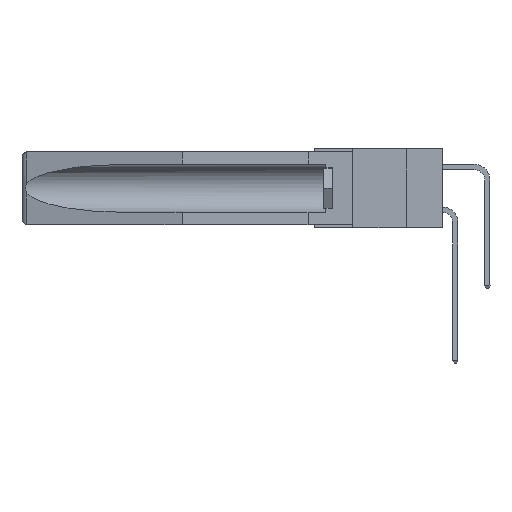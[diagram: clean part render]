
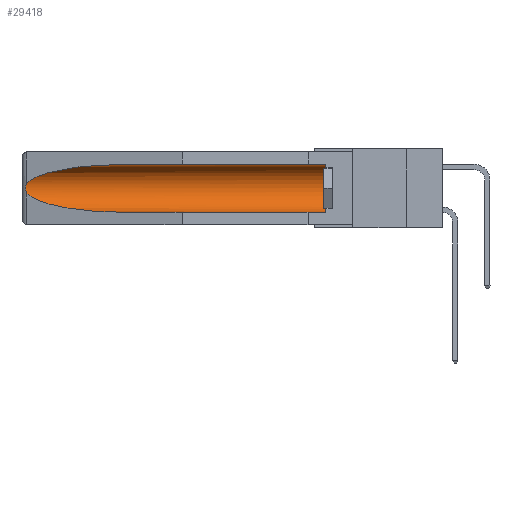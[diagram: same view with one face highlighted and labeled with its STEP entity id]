
A CAD part, left-side view. The second image highlights one B-rep face of the part: STEP entity #29418.
In plain terms, the highlighted cylindrical face has radius 2.857 mm (diameter 5.715 mm), a partial arc.
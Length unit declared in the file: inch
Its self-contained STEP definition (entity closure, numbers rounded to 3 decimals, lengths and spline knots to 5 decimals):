
#142 = EDGE_CURVE ( 'NONE', #16310, #8320, #24778, .T. ) ;
#195 = CARTESIAN_POINT ( 'NONE',  ( 0.21114, 1.30732, -0.059 ) ) ;
#409 = DIRECTION ( 'NONE',  ( 0., 0., 1. ) ) ;
#1260 = ORIENTED_EDGE ( 'NONE', *, *, #14060, .T. ) ;
#1483 = VERTEX_POINT ( 'NONE', #27589 ) ;
#1517 = CARTESIAN_POINT ( 'NONE',  ( 0.26537, 1.52718, -0.14972 ) ) ;
#1583 = DIRECTION ( 'NONE',  ( 0., 0., 1. ) ) ;
#1936 = CARTESIAN_POINT ( 'NONE',  ( 0.155, -0.30754, -0.284 ) ) ;
#1953 = CARTESIAN_POINT ( 'NONE',  ( 0.26537, 1.52718, -0.19328 ) ) ;
#2326 = VERTEX_POINT ( 'NONE', #5657 ) ;
#2421 = CARTESIAN_POINT ( 'NONE',  ( 0.155, -0.30754, -0.1715 ) ) ;
#5568 = CYLINDRICAL_SURFACE ( 'NONE', #19323, 0.1125 ) ;
#5657 = CARTESIAN_POINT ( 'NONE',  ( 0.155, 1.07973, -0.059 ) ) ;
#6466 = CARTESIAN_POINT ( 'NONE',  ( 0.25451, 1.48313, -0.09465 ) ) ;
#7957 = EDGE_CURVE ( 'NONE', #2326, #8256, #28995, .T. ) ;
#8209 = DIRECTION ( 'NONE',  ( 0., 1., 0. ) ) ;
#8256 = VERTEX_POINT ( 'NONE', #28920 ) ;
#8320 = VERTEX_POINT ( 'NONE', #12853 ) ;
#8803 = CARTESIAN_POINT ( 'NONE',  ( 0.2675, 1.53308, -0.17534 ) ) ;
#8817 = EDGE_CURVE ( 'NONE', #27200, #2326, #30827, .T. ) ;
#8905 = DIRECTION ( 'NONE',  ( 0., 1., 0. ) ) ;
#9609 = LINE ( 'NONE', #1936, #17907 ) ;
#9870 = DIRECTION ( 'NONE',  ( 0., 1., 0. ) ) ;
#10989 = EDGE_CURVE ( 'NONE', #1483, #27200, #17435, .T. ) ;
#10995 = CARTESIAN_POINT ( 'NONE',  ( 0.26655, 1.53094, -0.18657 ) ) ;
#11967 = FACE_OUTER_BOUND ( 'NONE', #29376, .T. ) ;
#12731 = CARTESIAN_POINT ( 'NONE',  ( 0.155, -0.30754, -0.059 ) ) ;
#12853 = CARTESIAN_POINT ( 'NONE',  ( 0.155, 1.07973, -0.284 ) ) ;
#14060 = EDGE_CURVE ( 'NONE', #8256, #16310, #20357, .T. ) ;
#15613 = CARTESIAN_POINT ( 'NONE',  ( 0.2673, 1.53269, -0.17917 ) ) ;
#15722 = CARTESIAN_POINT ( 'NONE',  ( 0.26597, 1.52961, -0.15275 ) ) ;
#16310 = VERTEX_POINT ( 'NONE', #1953 ) ;
#16503 = ORIENTED_EDGE ( 'NONE', *, *, #7957, .T. ) ;
#17119 = CARTESIAN_POINT ( 'NONE',  ( 0.155, 1.07973, -0.284 ) ) ;
#17360 = AXIS2_PLACEMENT_3D ( 'NONE', #20647, #27847, #1583 ) ;
#17435 = CIRCLE ( 'NONE', #17360, 0.1125 ) ;
#17907 = VECTOR ( 'NONE', #8905, 39.37008 ) ;
#18257 = CARTESIAN_POINT ( 'NONE',  ( 0.26537, 1.52718, -0.19328 ) ) ;
#18351 = ORIENTED_EDGE ( 'NONE', *, *, #10989, .T. ) ;
#18420 = VECTOR ( 'NONE', #8209, 39.37008 ) ;
#19200 = CARTESIAN_POINT ( 'NONE',  ( 0.155, 0.126, -0.059 ) ) ;
#19323 = AXIS2_PLACEMENT_3D ( 'NONE', #2421, #9870, #409 ) ;
#19757 = CARTESIAN_POINT ( 'NONE',  ( 0.25451, 1.48313, -0.24835 ) ) ;
#20357 = B_SPLINE_CURVE_WITH_KNOTS ( 'NONE', 3,
 ( #1517, #15722, #20787, #25488, #25391, #8803, #15613, #10995, #25594, #18257 ),
 .UNSPECIFIED., .F., .F.,
 ( 4, 2, 2, 2, 4 ),
 ( 0., 0.00029, 0.00058, 0.00087, 0.00117 ),
 .UNSPECIFIED. ) ;
#20647 = CARTESIAN_POINT ( 'NONE',  ( 0.155, 0.126, -0.1715 ) ) ;
#20650 = ORIENTED_EDGE ( 'NONE', *, *, #8817, .T. ) ;
#20787 = CARTESIAN_POINT ( 'NONE',  ( 0.26654, 1.53092, -0.15636 ) ) ;
#22183 = CARTESIAN_POINT ( 'NONE',  ( 0.21114, 1.30732, -0.284 ) ) ;
#23546 = EDGE_CURVE ( 'NONE', #1483, #8320, #9609, .T. ) ;
#24778 =( BOUNDED_CURVE ( )  B_SPLINE_CURVE ( 3, ( #25849, #19757, #22183, #17119 ),
 .UNSPECIFIED., .F., .F. ) 
 B_SPLINE_CURVE_WITH_KNOTS ( ( 4, 4 ),
 ( 0.1948, 1.5708 ),
 .UNSPECIFIED. ) 
 CURVE ( )  GEOMETRIC_REPRESENTATION_ITEM ( )  RATIONAL_B_SPLINE_CURVE ( ( 1., 0.848, 0.848, 1. ) ) 
 REPRESENTATION_ITEM ( '' )  );
#25391 = CARTESIAN_POINT ( 'NONE',  ( 0.2675, 1.53308, -0.16763 ) ) ;
#25488 = CARTESIAN_POINT ( 'NONE',  ( 0.2673, 1.5327, -0.16383 ) ) ;
#25594 = CARTESIAN_POINT ( 'NONE',  ( 0.26597, 1.5296, -0.19026 ) ) ;
#25849 = CARTESIAN_POINT ( 'NONE',  ( 0.26537, 1.52718, -0.19328 ) ) ;
#26239 = CARTESIAN_POINT ( 'NONE',  ( 0.155, 1.07973, -0.059 ) ) ;
#27200 = VERTEX_POINT ( 'NONE', #19200 ) ;
#27589 = CARTESIAN_POINT ( 'NONE',  ( 0.155, 0.126, -0.284 ) ) ;
#27847 = DIRECTION ( 'NONE',  ( 0., -1., 0. ) ) ;
#28621 = ORIENTED_EDGE ( 'NONE', *, *, #142, .T. ) ;
#28920 = CARTESIAN_POINT ( 'NONE',  ( 0.26537, 1.52718, -0.14972 ) ) ;
#28995 =( BOUNDED_CURVE ( )  B_SPLINE_CURVE ( 3, ( #26239, #195, #6466, #31106 ),
 .UNSPECIFIED., .F., .F. ) 
 B_SPLINE_CURVE_WITH_KNOTS ( ( 4, 4 ),
 ( 4.71239, 6.08839 ),
 .UNSPECIFIED. ) 
 CURVE ( )  GEOMETRIC_REPRESENTATION_ITEM ( )  RATIONAL_B_SPLINE_CURVE ( ( 1., 0.848, 0.848, 1. ) ) 
 REPRESENTATION_ITEM ( '' )  );
#29376 = EDGE_LOOP ( 'NONE', ( #16503, #1260, #28621, #29912, #18351, #20650 ) ) ;
#29418 = ADVANCED_FACE ( 'NONE', ( #11967 ), #5568, .F. ) ;
#29912 = ORIENTED_EDGE ( 'NONE', *, *, #23546, .F. ) ;
#30827 = LINE ( 'NONE', #12731, #18420 ) ;
#31106 = CARTESIAN_POINT ( 'NONE',  ( 0.26537, 1.52718, -0.14972 ) ) ;
